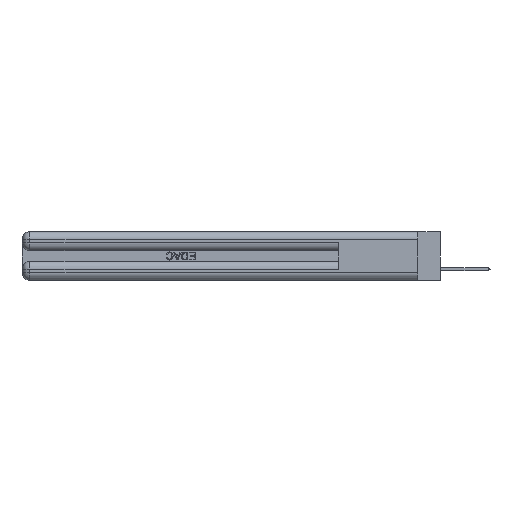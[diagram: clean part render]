
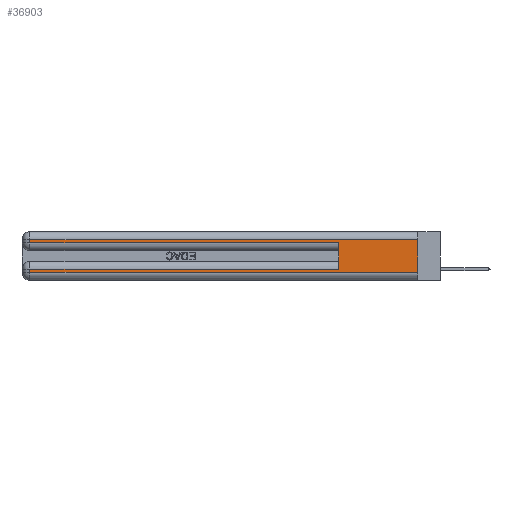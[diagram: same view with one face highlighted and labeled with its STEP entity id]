
A CAD part, left-side view. The second image highlights one B-rep face of the part: STEP entity #36903.
In plain terms, the highlighted planar face has unit normal (-1, 0, 0).
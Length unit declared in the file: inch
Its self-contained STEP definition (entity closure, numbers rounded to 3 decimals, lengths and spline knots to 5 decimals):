
#224 = LINE ( 'NONE', #35962, #19499 ) ;
#1021 = VECTOR ( 'NONE', #20577, 39.37008 ) ;
#1290 = CARTESIAN_POINT ( 'NONE',  ( 0., 0., 0.06 ) ) ;
#3362 = DIRECTION ( 'NONE',  ( 0., 0., -1. ) ) ;
#3473 = DIRECTION ( 'NONE',  ( 1., 0., 0. ) ) ;
#3871 = CARTESIAN_POINT ( 'NONE',  ( 0., 0.6, 0.285 ) ) ;
#5273 = EDGE_CURVE ( 'NONE', #40180, #35080, #224, .T. ) ;
#5522 = VECTOR ( 'NONE', #26944, 39.37008 ) ;
#5925 = CARTESIAN_POINT ( 'NONE',  ( 0., 0.6, 0.085 ) ) ;
#6501 = VERTEX_POINT ( 'NONE', #5925 ) ;
#7654 = ORIENTED_EDGE ( 'NONE', *, *, #30474, .T. ) ;
#11446 = CARTESIAN_POINT ( 'NONE',  ( 0., 2.94, 0.06 ) ) ;
#11461 = PLANE ( 'NONE',  #48504 ) ;
#11738 = VECTOR ( 'NONE', #43879, 39.37008 ) ;
#12228 = ORIENTED_EDGE ( 'NONE', *, *, #39302, .T. ) ;
#13190 = ORIENTED_EDGE ( 'NONE', *, *, #29004, .T. ) ;
#13442 = ORIENTED_EDGE ( 'NONE', *, *, #41585, .T. ) ;
#13826 = VERTEX_POINT ( 'NONE', #11446 ) ;
#14597 = VECTOR ( 'NONE', #54811, 39.37008 ) ;
#15112 = DIRECTION ( 'NONE',  ( 0., 0., -1. ) ) ;
#15205 = CARTESIAN_POINT ( 'NONE',  ( 0., 0., 0.085 ) ) ;
#15772 = DIRECTION ( 'NONE',  ( 0., 0., -1. ) ) ;
#18584 = ORIENTED_EDGE ( 'NONE', *, *, #39606, .T. ) ;
#18816 = LINE ( 'NONE', #31446, #5522 ) ;
#19499 = VECTOR ( 'NONE', #15112, 39.37008 ) ;
#20577 = DIRECTION ( 'NONE',  ( 0., -1., 0. ) ) ;
#24467 = CARTESIAN_POINT ( 'NONE',  ( 0., 2.94, 0.37 ) ) ;
#24590 = CARTESIAN_POINT ( 'NONE',  ( 0., 2.94, 0.37 ) ) ;
#26497 = VERTEX_POINT ( 'NONE', #3871 ) ;
#26944 = DIRECTION ( 'NONE',  ( 0., 0., 1. ) ) ;
#27788 = FACE_OUTER_BOUND ( 'NONE', #38916, .T. ) ;
#29004 = EDGE_CURVE ( 'NONE', #40180, #45792, #43462, .T. ) ;
#29854 = CARTESIAN_POINT ( 'NONE',  ( 0., 2.94, 0.085 ) ) ;
#30474 = EDGE_CURVE ( 'NONE', #45792, #45735, #50657, .T. ) ;
#31446 = CARTESIAN_POINT ( 'NONE',  ( 0., 0.6, 0.145 ) ) ;
#31551 = ORIENTED_EDGE ( 'NONE', *, *, #5273, .F. ) ;
#32287 = VECTOR ( 'NONE', #47447, 39.37008 ) ;
#35080 = VERTEX_POINT ( 'NONE', #47559 ) ;
#35962 = CARTESIAN_POINT ( 'NONE',  ( 0., 0., 0.37 ) ) ;
#36184 = LINE ( 'NONE', #45882, #1021 ) ;
#36903 = ADVANCED_FACE ( 'NONE', ( #27788 ), #11461, .F. ) ;
#38916 = EDGE_LOOP ( 'NONE', ( #31551, #13190, #7654, #13442, #41495, #12228, #18584, #44112 ) ) ;
#39047 = VECTOR ( 'NONE', #52383, 39.37008 ) ;
#39302 = EDGE_CURVE ( 'NONE', #6501, #51245, #41135, .T. ) ;
#39606 = EDGE_CURVE ( 'NONE', #51245, #13826, #42383, .T. ) ;
#40180 = VERTEX_POINT ( 'NONE', #49703 ) ;
#41135 = LINE ( 'NONE', #15205, #39047 ) ;
#41495 = ORIENTED_EDGE ( 'NONE', *, *, #48739, .F. ) ;
#41585 = EDGE_CURVE ( 'NONE', #45735, #26497, #36184, .T. ) ;
#42383 = LINE ( 'NONE', #24590, #14597 ) ;
#43462 = LINE ( 'NONE', #47098, #32287 ) ;
#43879 = DIRECTION ( 'NONE',  ( 0., -1., 0. ) ) ;
#44112 = ORIENTED_EDGE ( 'NONE', *, *, #46766, .T. ) ;
#44116 = LINE ( 'NONE', #1290, #11738 ) ;
#45510 = CARTESIAN_POINT ( 'NONE',  ( 0., 0., 0.37 ) ) ;
#45735 = VERTEX_POINT ( 'NONE', #53344 ) ;
#45792 = VERTEX_POINT ( 'NONE', #53924 ) ;
#45882 = CARTESIAN_POINT ( 'NONE',  ( 0., 0., 0.285 ) ) ;
#46766 = EDGE_CURVE ( 'NONE', #13826, #35080, #44116, .T. ) ;
#47098 = CARTESIAN_POINT ( 'NONE',  ( 0., 0., 0.31 ) ) ;
#47447 = DIRECTION ( 'NONE',  ( 0., 1., 0. ) ) ;
#47559 = CARTESIAN_POINT ( 'NONE',  ( 0., 0., 0.06 ) ) ;
#48504 = AXIS2_PLACEMENT_3D ( 'NONE', #45510, #3473, #15772 ) ;
#48739 = EDGE_CURVE ( 'NONE', #6501, #26497, #18816, .T. ) ;
#49703 = CARTESIAN_POINT ( 'NONE',  ( 0., 0., 0.31 ) ) ;
#50657 = LINE ( 'NONE', #24467, #53975 ) ;
#51245 = VERTEX_POINT ( 'NONE', #29854 ) ;
#52383 = DIRECTION ( 'NONE',  ( 0., 1., 0. ) ) ;
#53344 = CARTESIAN_POINT ( 'NONE',  ( 0., 2.94, 0.285 ) ) ;
#53924 = CARTESIAN_POINT ( 'NONE',  ( 0., 2.94, 0.31 ) ) ;
#53975 = VECTOR ( 'NONE', #3362, 39.37008 ) ;
#54811 = DIRECTION ( 'NONE',  ( 0., 0., -1. ) ) ;
